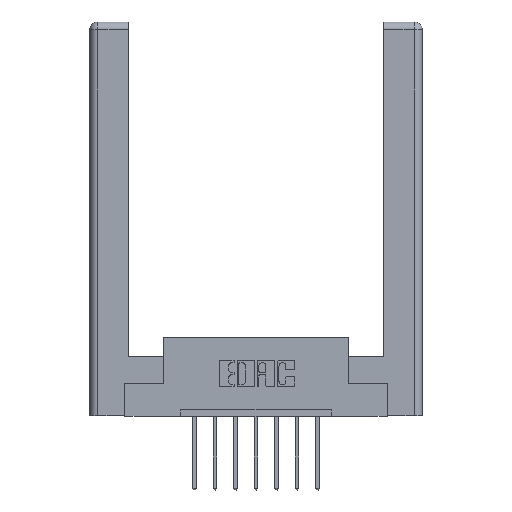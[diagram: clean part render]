
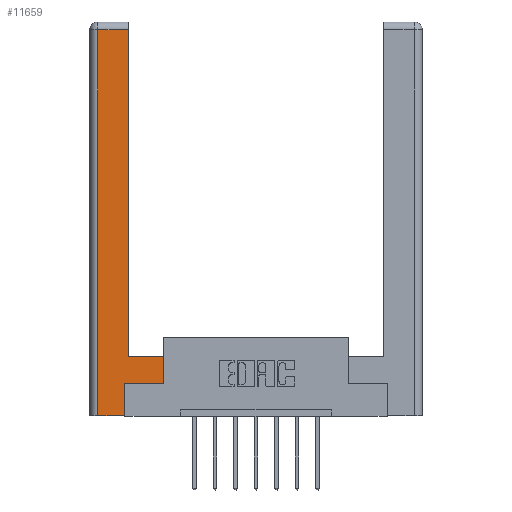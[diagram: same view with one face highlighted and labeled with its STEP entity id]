
A CAD part, top view. The second image highlights one B-rep face of the part: STEP entity #11659.
In plain terms, the highlighted planar face has unit normal (0, 0, 1).
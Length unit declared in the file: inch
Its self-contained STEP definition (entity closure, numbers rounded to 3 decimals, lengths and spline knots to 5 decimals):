
#111 = CARTESIAN_POINT ( 'NONE',  ( 0.265, 0., 0. ) ) ;
#116 = VECTOR ( 'NONE', #387, 39.37008 ) ;
#145 = LINE ( 'NONE', #503, #7777 ) ;
#185 = ORIENTED_EDGE ( 'NONE', *, *, #7021, .T. ) ;
#206 = EDGE_CURVE ( 'NONE', #3735, #5716, #1290, .T. ) ;
#387 = DIRECTION ( 'NONE',  ( -1., 0., 0. ) ) ;
#503 = CARTESIAN_POINT ( 'NONE',  ( 0.265, 0.245, 0. ) ) ;
#516 = VERTEX_POINT ( 'NONE', #5870 ) ;
#598 = ORIENTED_EDGE ( 'NONE', *, *, #9999, .T. ) ;
#646 = VERTEX_POINT ( 'NONE', #5117 ) ;
#881 = CARTESIAN_POINT ( 'NONE',  ( 0.0615, 2.94, 0. ) ) ;
#906 = VECTOR ( 'NONE', #8698, 39.37008 ) ;
#920 = FACE_OUTER_BOUND ( 'NONE', #995, .T. ) ;
#971 = CARTESIAN_POINT ( 'NONE',  ( 0.565, 0.245, 0. ) ) ;
#995 = EDGE_LOOP ( 'NONE', ( #10554, #2699, #6038, #4568, #185, #9806, #598, #2330 ) ) ;
#998 = CARTESIAN_POINT ( 'NONE',  ( 0.0615, 0., 0. ) ) ;
#1029 = VERTEX_POINT ( 'NONE', #6964 ) ;
#1107 = DIRECTION ( 'NONE',  ( -1., 0., 0. ) ) ;
#1290 = LINE ( 'NONE', #1447, #116 ) ;
#1447 = CARTESIAN_POINT ( 'NONE',  ( 0.295, 0.45, 0. ) ) ;
#1682 = EDGE_CURVE ( 'NONE', #1029, #5513, #5313, .T. ) ;
#1999 = DIRECTION ( 'NONE',  ( 1., 0., 0. ) ) ;
#2135 = VECTOR ( 'NONE', #5272, 39.37008 ) ;
#2156 = VERTEX_POINT ( 'NONE', #111 ) ;
#2330 = ORIENTED_EDGE ( 'NONE', *, *, #206, .T. ) ;
#2676 = VECTOR ( 'NONE', #1999, 39.37008 ) ;
#2699 = ORIENTED_EDGE ( 'NONE', *, *, #10876, .T. ) ;
#3553 = CARTESIAN_POINT ( 'NONE',  ( 0.565, 0.45, 0. ) ) ;
#3609 = VERTEX_POINT ( 'NONE', #4794 ) ;
#3702 = CARTESIAN_POINT ( 'NONE',  ( 0.295, 3., 0. ) ) ;
#3735 = VERTEX_POINT ( 'NONE', #10071 ) ;
#4568 = ORIENTED_EDGE ( 'NONE', *, *, #9683, .T. ) ;
#4794 = CARTESIAN_POINT ( 'NONE',  ( 0.565, 0.245, 0. ) ) ;
#5117 = CARTESIAN_POINT ( 'NONE',  ( 0.265, 0.245, 0. ) ) ;
#5272 = DIRECTION ( 'NONE',  ( 1., 0., 0. ) ) ;
#5313 = LINE ( 'NONE', #998, #5908 ) ;
#5513 = VERTEX_POINT ( 'NONE', #6373 ) ;
#5581 = LINE ( 'NONE', #7488, #2135 ) ;
#5716 = VERTEX_POINT ( 'NONE', #11271 ) ;
#5870 = CARTESIAN_POINT ( 'NONE',  ( 0.295, 2.94, 0. ) ) ;
#5900 = DIRECTION ( 'NONE',  ( 0., 0., -1. ) ) ;
#5908 = VECTOR ( 'NONE', #8682, 39.37008 ) ;
#6038 = ORIENTED_EDGE ( 'NONE', *, *, #1682, .T. ) ;
#6373 = CARTESIAN_POINT ( 'NONE',  ( 0.0615, 0., 0. ) ) ;
#6435 = LINE ( 'NONE', #971, #2676 ) ;
#6964 = CARTESIAN_POINT ( 'NONE',  ( 0.0615, 2.94, 0. ) ) ;
#7021 = EDGE_CURVE ( 'NONE', #2156, #646, #145, .T. ) ;
#7283 = DIRECTION ( 'NONE',  ( 0., 1., 0. ) ) ;
#7488 = CARTESIAN_POINT ( 'NONE',  ( 0.265, 0., 0. ) ) ;
#7647 = LINE ( 'NONE', #3702, #906 ) ;
#7705 = DIRECTION ( 'NONE',  ( -1., 0., 0. ) ) ;
#7777 = VECTOR ( 'NONE', #8006, 39.37008 ) ;
#8006 = DIRECTION ( 'NONE',  ( 0., 1., 0. ) ) ;
#8314 = LINE ( 'NONE', #3553, #12193 ) ;
#8682 = DIRECTION ( 'NONE',  ( 0., -1., 0. ) ) ;
#8698 = DIRECTION ( 'NONE',  ( 0., 1., 0. ) ) ;
#9683 = EDGE_CURVE ( 'NONE', #5513, #2156, #5581, .T. ) ;
#9806 = ORIENTED_EDGE ( 'NONE', *, *, #12231, .T. ) ;
#9813 = PLANE ( 'NONE',  #12140 ) ;
#9999 = EDGE_CURVE ( 'NONE', #3609, #3735, #8314, .T. ) ;
#10071 = CARTESIAN_POINT ( 'NONE',  ( 0.565, 0.45, 0. ) ) ;
#10554 = ORIENTED_EDGE ( 'NONE', *, *, #12126, .T. ) ;
#10784 = CARTESIAN_POINT ( 'NONE',  ( 0., 0., 0. ) ) ;
#10876 = EDGE_CURVE ( 'NONE', #516, #1029, #12031, .T. ) ;
#11271 = CARTESIAN_POINT ( 'NONE',  ( 0.295, 0.45, 0. ) ) ;
#11659 = ADVANCED_FACE ( 'NONE', ( #920 ), #9813, .F. ) ;
#12031 = LINE ( 'NONE', #881, #12048 ) ;
#12048 = VECTOR ( 'NONE', #7705, 39.37008 ) ;
#12126 = EDGE_CURVE ( 'NONE', #5716, #516, #7647, .T. ) ;
#12140 = AXIS2_PLACEMENT_3D ( 'NONE', #10784, #5900, #1107 ) ;
#12193 = VECTOR ( 'NONE', #7283, 39.37008 ) ;
#12231 = EDGE_CURVE ( 'NONE', #646, #3609, #6435, .T. ) ;
